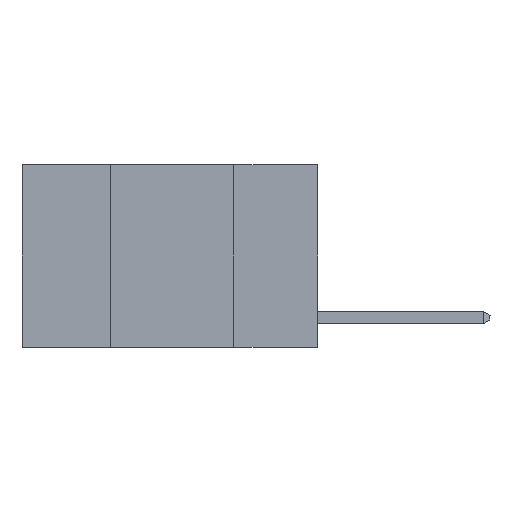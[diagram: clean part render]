
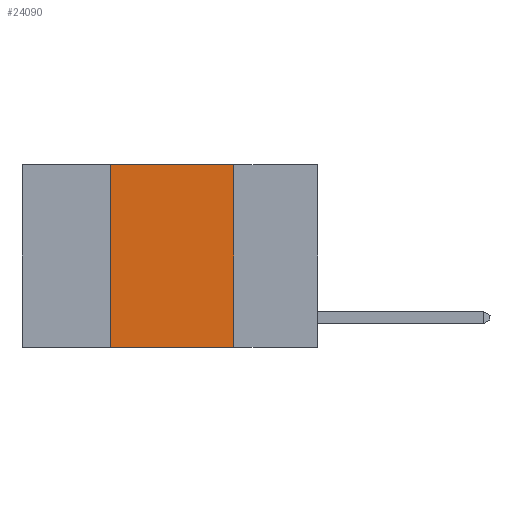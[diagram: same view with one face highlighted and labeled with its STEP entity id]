
A CAD part, left-side view. The second image highlights one B-rep face of the part: STEP entity #24090.
In plain terms, the highlighted planar face has unit normal (-1, 0, 0).
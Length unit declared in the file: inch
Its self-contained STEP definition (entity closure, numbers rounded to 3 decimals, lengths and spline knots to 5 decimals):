
#1047 = EDGE_CURVE ( 'NONE', #2680, #10308, #9264, .T. ) ;
#1125 = ORIENTED_EDGE ( 'NONE', *, *, #1047, .F. ) ;
#1935 = DIRECTION ( 'NONE',  ( 1., 0., 0. ) ) ;
#2190 = EDGE_CURVE ( 'NONE', #14041, #19854, #6529, .T. ) ;
#2680 = VERTEX_POINT ( 'NONE', #19465 ) ;
#2689 = CARTESIAN_POINT ( 'NONE',  ( 0., 0.42, 0. ) ) ;
#3225 = AXIS2_PLACEMENT_3D ( 'NONE', #15612, #1935, #5904 ) ;
#3324 = VECTOR ( 'NONE', #12933, 39.37008 ) ;
#4682 = EDGE_CURVE ( 'NONE', #14041, #10308, #18399, .T. ) ;
#5904 = DIRECTION ( 'NONE',  ( 0., 0., -1. ) ) ;
#6100 = VECTOR ( 'NONE', #20700, 39.37008 ) ;
#6529 = LINE ( 'NONE', #18519, #19561 ) ;
#6748 = ORIENTED_EDGE ( 'NONE', *, *, #12203, .F. ) ;
#7044 = DIRECTION ( 'NONE',  ( 0., -1., 0. ) ) ;
#7164 = CARTESIAN_POINT ( 'NONE',  ( 0., 0.6, -0.37 ) ) ;
#7973 = CARTESIAN_POINT ( 'NONE',  ( 0., 0.42, -0.37 ) ) ;
#7988 = CARTESIAN_POINT ( 'NONE',  ( 0., 0.17, -0.37 ) ) ;
#8921 = ORIENTED_EDGE ( 'NONE', *, *, #4682, .T. ) ;
#9218 = CARTESIAN_POINT ( 'NONE',  ( 0., 0.6, 0. ) ) ;
#9264 = LINE ( 'NONE', #18835, #3324 ) ;
#10308 = VERTEX_POINT ( 'NONE', #7988 ) ;
#12203 = EDGE_CURVE ( 'NONE', #19854, #2680, #20703, .T. ) ;
#12933 = DIRECTION ( 'NONE',  ( 0., 0., -1. ) ) ;
#14041 = VERTEX_POINT ( 'NONE', #7973 ) ;
#15612 = CARTESIAN_POINT ( 'NONE',  ( 0., 0.6, 0. ) ) ;
#16583 = DIRECTION ( 'NONE',  ( 0., 0., 1. ) ) ;
#18399 = LINE ( 'NONE', #7164, #6100 ) ;
#18519 = CARTESIAN_POINT ( 'NONE',  ( 0., 0.42, 0. ) ) ;
#18835 = CARTESIAN_POINT ( 'NONE',  ( 0., 0.17, 0. ) ) ;
#18859 = EDGE_LOOP ( 'NONE', ( #1125, #6748, #20328, #8921 ) ) ;
#19465 = CARTESIAN_POINT ( 'NONE',  ( 0., 0.17, 0. ) ) ;
#19561 = VECTOR ( 'NONE', #16583, 39.37008 ) ;
#19854 = VERTEX_POINT ( 'NONE', #2689 ) ;
#20328 = ORIENTED_EDGE ( 'NONE', *, *, #2190, .F. ) ;
#20700 = DIRECTION ( 'NONE',  ( 0., -1., 0. ) ) ;
#20703 = LINE ( 'NONE', #9218, #24683 ) ;
#23168 = FACE_OUTER_BOUND ( 'NONE', #18859, .T. ) ;
#23430 = PLANE ( 'NONE',  #3225 ) ;
#24090 = ADVANCED_FACE ( 'NONE', ( #23168 ), #23430, .F. ) ;
#24683 = VECTOR ( 'NONE', #7044, 39.37008 ) ;
